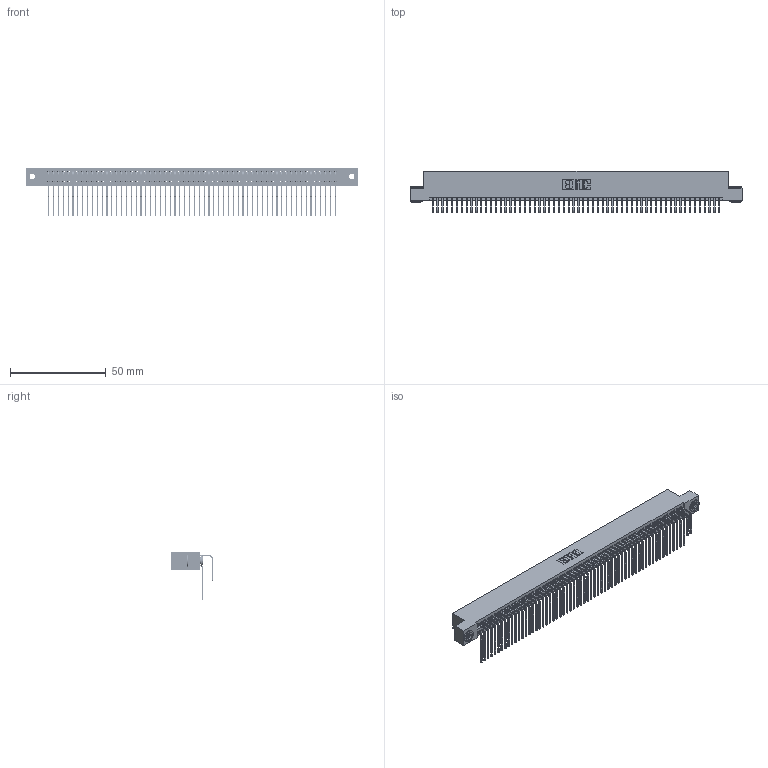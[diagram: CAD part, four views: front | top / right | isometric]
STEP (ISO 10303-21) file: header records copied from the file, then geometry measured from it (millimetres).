
FILE_DESCRIPTION (( 'STEP AP203' ), '1' );
FILE_NAME ('845-120-558-203.STEP', '2018-11-21T06:13:38', ( '' ), ( '' ), 'SwSTEP 2.0', 'SolidWorks 2016', '' );
FILE_SCHEMA (( 'CONFIG_CONTROL_DESIGN' ));
Length unit declared in the file: inch
Products named in the file (5): 845 Part_Flush Mounting Lugs - 0.156 Dia-TH; 345-292-001_558 559 Tail - 1; 345-292-001_558 Tail - 2; 345-250-002_345-250-002-102; 845-120-558-203
Assembly tree (123 placements, depth 2):
  845-120-558-203
    845 Part_Flush Mounting Lugs - 0.156 Dia-TH
    345-292-001_558 559 Tail - 1  x60
    345-292-001_558 Tail - 2  x60
    345-250-002_345-250-002-102  x2
Bounding box: 173.61 x 21.83 x 25.53 mm (x, y, z)
Volume: 17743.3 mm3; surface area: 30036.2 mm2
Topology: 123 solids, 123 shells, 6404 faces, 19017 edges, 12514 vertices
Faces by surface type: plane 4290, cylinder 2106, cone 8
Entity records: 46956 total; most frequent: CARTESIAN_POINT 7874, ORIENTED_EDGE 7750, DIRECTION 6925, EDGE_CURVE 3875, LINE 3439, VECTOR 3439, VERTEX_POINT 2578, AXIS2_PLACEMENT_3D 1743
